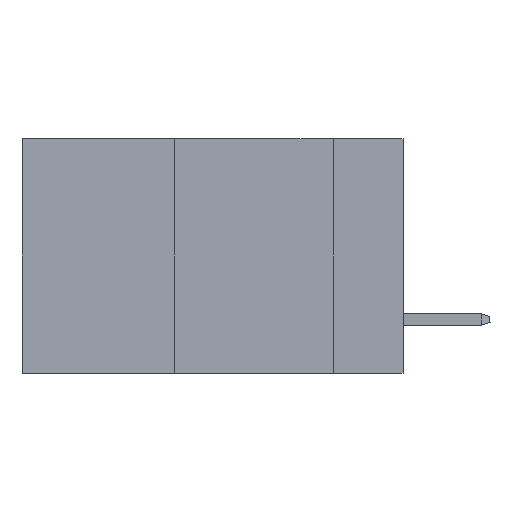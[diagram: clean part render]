
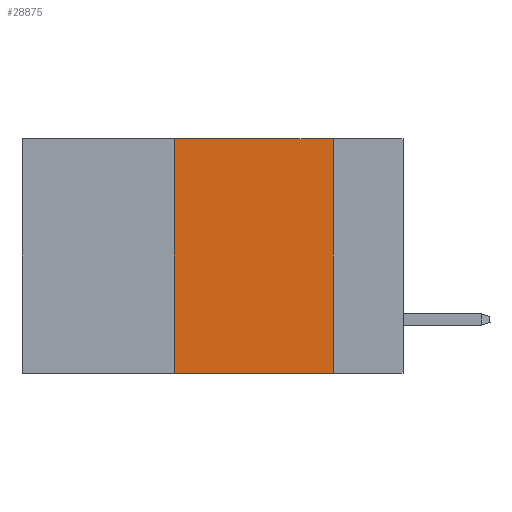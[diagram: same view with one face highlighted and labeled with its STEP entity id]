
A CAD part, left-side view. The second image highlights one B-rep face of the part: STEP entity #28875.
In plain terms, the highlighted planar face has unit normal (-1, 0, 0).
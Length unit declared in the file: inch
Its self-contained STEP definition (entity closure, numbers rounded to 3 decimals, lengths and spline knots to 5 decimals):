
#1074 = VERTEX_POINT ( 'NONE', #16071 ) ;
#1136 = ORIENTED_EDGE ( 'NONE', *, *, #16153, .F. ) ;
#1608 = CARTESIAN_POINT ( 'NONE',  ( 0., 0.36, 0. ) ) ;
#1895 = DIRECTION ( 'NONE',  ( 0., -1., 0. ) ) ;
#1965 = VERTEX_POINT ( 'NONE', #28922 ) ;
#3430 = VECTOR ( 'NONE', #31939, 39.37008 ) ;
#3764 = CARTESIAN_POINT ( 'NONE',  ( 0., 0.11, -0.37 ) ) ;
#5061 = CARTESIAN_POINT ( 'NONE',  ( 0., 0.6, 0. ) ) ;
#5212 = LINE ( 'NONE', #25015, #32157 ) ;
#5789 = AXIS2_PLACEMENT_3D ( 'NONE', #5061, #12130, #7371 ) ;
#7371 = DIRECTION ( 'NONE',  ( 0., 0., -1. ) ) ;
#7515 = DIRECTION ( 'NONE',  ( 0., 0., -1. ) ) ;
#10799 = LINE ( 'NONE', #21249, #27546 ) ;
#11146 = EDGE_CURVE ( 'NONE', #28577, #1965, #26669, .T. ) ;
#12130 = DIRECTION ( 'NONE',  ( 1., 0., 0. ) ) ;
#12481 = EDGE_CURVE ( 'NONE', #1965, #25109, #5212, .T. ) ;
#13916 = DIRECTION ( 'NONE',  ( 0., 0., 1. ) ) ;
#14238 = ORIENTED_EDGE ( 'NONE', *, *, #12481, .F. ) ;
#14761 = FACE_OUTER_BOUND ( 'NONE', #26149, .T. ) ;
#14906 = ORIENTED_EDGE ( 'NONE', *, *, #11146, .F. ) ;
#16071 = CARTESIAN_POINT ( 'NONE',  ( 0., 0.36, -0.37 ) ) ;
#16153 = EDGE_CURVE ( 'NONE', #1074, #28577, #19481, .T. ) ;
#16501 = EDGE_CURVE ( 'NONE', #1074, #25109, #10799, .T. ) ;
#18211 = CARTESIAN_POINT ( 'NONE',  ( 0., 0.36, 0. ) ) ;
#19481 = LINE ( 'NONE', #1608, #23854 ) ;
#21249 = CARTESIAN_POINT ( 'NONE',  ( 0., 0.6, -0.37 ) ) ;
#23854 = VECTOR ( 'NONE', #13916, 39.37008 ) ;
#25015 = CARTESIAN_POINT ( 'NONE',  ( 0., 0.11, 0. ) ) ;
#25109 = VERTEX_POINT ( 'NONE', #3764 ) ;
#26149 = EDGE_LOOP ( 'NONE', ( #14238, #14906, #1136, #26358 ) ) ;
#26358 = ORIENTED_EDGE ( 'NONE', *, *, #16501, .T. ) ;
#26669 = LINE ( 'NONE', #31616, #3430 ) ;
#27546 = VECTOR ( 'NONE', #1895, 39.37008 ) ;
#28577 = VERTEX_POINT ( 'NONE', #18211 ) ;
#28875 = ADVANCED_FACE ( 'NONE', ( #14761 ), #29819, .F. ) ;
#28922 = CARTESIAN_POINT ( 'NONE',  ( 0., 0.11, 0. ) ) ;
#29819 = PLANE ( 'NONE',  #5789 ) ;
#31616 = CARTESIAN_POINT ( 'NONE',  ( 0., 0.6, 0. ) ) ;
#31939 = DIRECTION ( 'NONE',  ( 0., -1., 0. ) ) ;
#32157 = VECTOR ( 'NONE', #7515, 39.37008 ) ;
